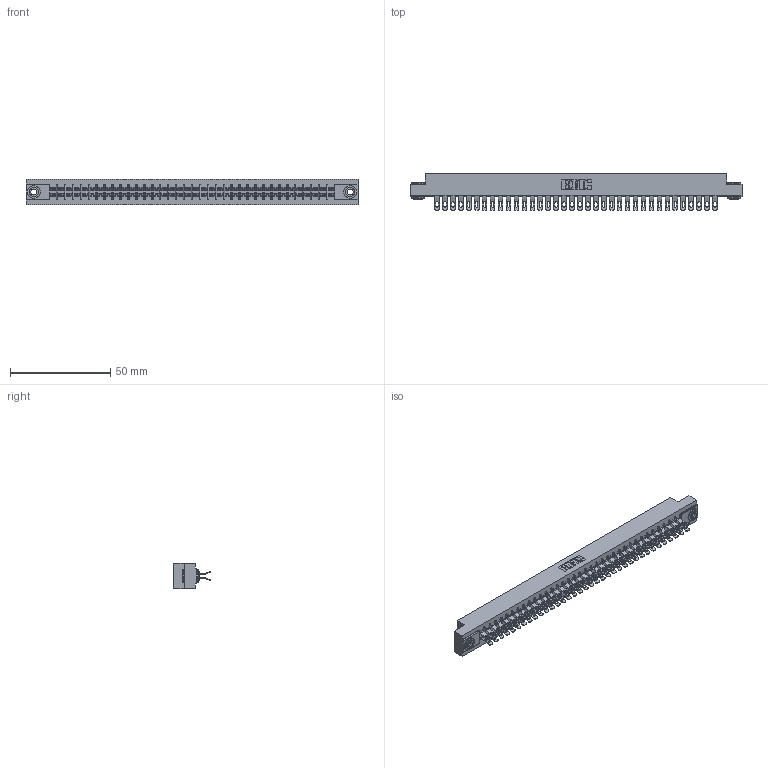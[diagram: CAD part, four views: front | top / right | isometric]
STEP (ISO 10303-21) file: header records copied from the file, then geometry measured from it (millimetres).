
FILE_DESCRIPTION (( 'STEP AP203' ), '1' );
FILE_NAME ('355-072-555-503.STEP', '2019-09-13T12:17:08', ( '' ), ( '' ), 'SwSTEP 2.0', 'SolidWorks 2016', '' );
FILE_SCHEMA (( 'CONFIG_CONTROL_DESIGN' ));
Length unit declared in the file: inch
Products named in the file (4): 355-072-555-503; 305 Part_.156 Dia; 305-290-001_555; 345-250-002_345-250-002-102
Assembly tree (75 placements, depth 2):
  355-072-555-503
    305 Part_.156 Dia
    305-290-001_555  x72
    345-250-002_345-250-002-102  x2
Bounding box: 165.66 x 18.41 x 12.7 mm (x, y, z)
Volume: 16962.1 mm3; surface area: 23846.2 mm2
Topology: 75 solids, 75 shells, 4920 faces, 14648 edges, 9568 vertices
Faces by surface type: plane 2396, cylinder 2372, sphere 144, cone 8
Entity records: 41398 total; most frequent: CARTESIAN_POINT 6849, ORIENTED_EDGE 6780, DIRECTION 6640, EDGE_CURVE 3390, VECTOR 2706, LINE 2706, VERTEX_POINT 2160, AXIS2_PLACEMENT_3D 1967
